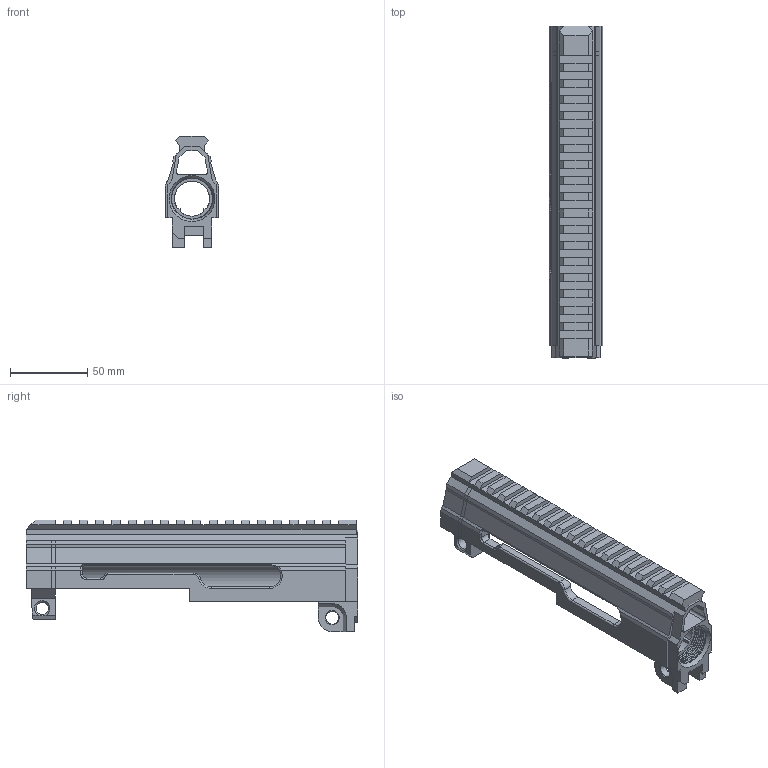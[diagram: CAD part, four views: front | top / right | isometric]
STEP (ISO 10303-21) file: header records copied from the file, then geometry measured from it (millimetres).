
FILE_DESCRIPTION(/* description */ (''),/* implementation_level */ '2;1');
FILE_NAME(/* name */ '522 Upper Reciever.step',/* time_stamp */ '2021-09-13T05:35:26-04:00',/* author */ (''),/* organization */ (''),/* preprocessor_version */ 'ST-DEVELOPER v18.1',/* originating_system */ 'Autodesk Translation Framework v10.10.0.1391',/* authorisation */ '');
FILE_SCHEMA (('AUTOMOTIVE_DESIGN { 1 0 10303 214 3 1 1 }'));
Length unit declared in the file: millimetre
Products named in the file (1): 522 Upper Reciever
Bounding box: 34.6 x 214.65 x 72.14 mm (x, y, z)
Volume: 153232.4 mm3; surface area: 71869.1 mm2
Topology: 3 solids, 3 shells, 307 faces, 861 edges, 555 vertices
Faces by surface type: plane 247, cylinder 41, cone 8, torus 6, bspline 5
Full cylindrical faces by diameter (mm): 8 x1, 8.3 x2, 22.75 x1, 26.526 x6, 28.208 x6
Entity records: 11913 total; most frequent: CARTESIAN_POINT 4021, ORIENTED_EDGE 1722, DIRECTION 1493, EDGE_CURVE 861, LINE 729, VECTOR 729, VERTEX_POINT 555, AXIS2_PLACEMENT_3D 382
